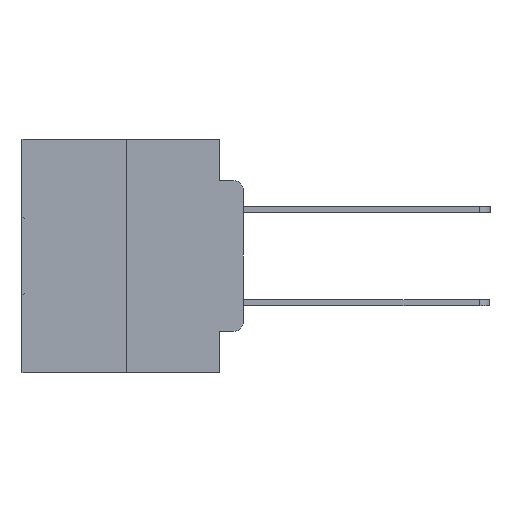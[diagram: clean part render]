
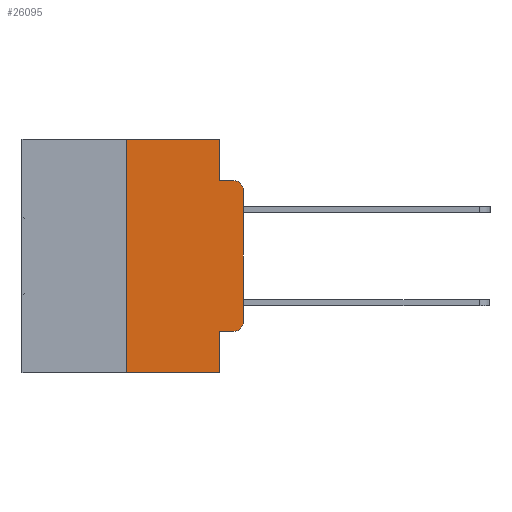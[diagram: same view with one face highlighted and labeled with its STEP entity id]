
A CAD part, left-side view. The second image highlights one B-rep face of the part: STEP entity #26095.
In plain terms, the highlighted planar face has unit normal (-1, 0, 0).
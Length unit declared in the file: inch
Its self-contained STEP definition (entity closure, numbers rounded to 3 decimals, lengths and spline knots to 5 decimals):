
#663 = LINE ( 'NONE', #30555, #26407 ) ;
#740 = ORIENTED_EDGE ( 'NONE', *, *, #30490, .F. ) ;
#1417 = CIRCLE ( 'NONE', #31994, 0.02 ) ;
#1953 = VERTEX_POINT ( 'NONE', #15396 ) ;
#2614 = VERTEX_POINT ( 'NONE', #27927 ) ;
#2710 = ORIENTED_EDGE ( 'NONE', *, *, #6122, .F. ) ;
#2886 = LINE ( 'NONE', #31540, #15412 ) ;
#2908 = VECTOR ( 'NONE', #31604, 39.37008 ) ;
#2981 = VECTOR ( 'NONE', #24101, 39.37008 ) ;
#4121 = EDGE_CURVE ( 'NONE', #15564, #19017, #8856, .T. ) ;
#4308 = DIRECTION ( 'NONE',  ( 1., 0., 0. ) ) ;
#4544 = EDGE_LOOP ( 'NONE', ( #15962, #8123, #16779, #740, #14441, #2710, #28045, #17174, #17570, #15645 ) ) ;
#4629 = LINE ( 'NONE', #19878, #29623 ) ;
#4911 = DIRECTION ( 'NONE',  ( 0., 0., -1. ) ) ;
#5365 = CARTESIAN_POINT ( 'NONE',  ( 0., 0., -0.1085 ) ) ;
#5631 = CARTESIAN_POINT ( 'NONE',  ( 0., 0.25, -0.5 ) ) ;
#6089 = LINE ( 'NONE', #9813, #25972 ) ;
#6122 = EDGE_CURVE ( 'NONE', #10830, #1953, #2886, .T. ) ;
#8123 = ORIENTED_EDGE ( 'NONE', *, *, #11843, .T. ) ;
#8293 = EDGE_CURVE ( 'NONE', #2614, #22981, #23102, .T. ) ;
#8492 = EDGE_CURVE ( 'NONE', #23985, #13070, #17676, .T. ) ;
#8856 = LINE ( 'NONE', #21541, #2981 ) ;
#9065 = CARTESIAN_POINT ( 'NONE',  ( 0., 0.051, 0. ) ) ;
#9229 = CARTESIAN_POINT ( 'NONE',  ( 0., 0.473, 0. ) ) ;
#9553 = DIRECTION ( 'NONE',  ( -1., 0., 0. ) ) ;
#9813 = CARTESIAN_POINT ( 'NONE',  ( 0., 0.473, 0. ) ) ;
#9939 = CARTESIAN_POINT ( 'NONE',  ( 0., 0.02, -0.1085 ) ) ;
#10414 = CIRCLE ( 'NONE', #11865, 0.02 ) ;
#10830 = VERTEX_POINT ( 'NONE', #5631 ) ;
#11491 = EDGE_CURVE ( 'NONE', #10830, #30007, #663, .T. ) ;
#11657 = CARTESIAN_POINT ( 'NONE',  ( 0., 0.051, 0. ) ) ;
#11843 = EDGE_CURVE ( 'NONE', #22981, #19017, #10414, .T. ) ;
#11865 = AXIS2_PLACEMENT_3D ( 'NONE', #9939, #27367, #12462 ) ;
#12462 = DIRECTION ( 'NONE',  ( 0., 0., -1. ) ) ;
#12673 = CARTESIAN_POINT ( 'NONE',  ( 0., 0.051, -0.0885 ) ) ;
#13070 = VERTEX_POINT ( 'NONE', #19602 ) ;
#14263 = PLANE ( 'NONE',  #26954 ) ;
#14441 = ORIENTED_EDGE ( 'NONE', *, *, #20208, .F. ) ;
#14484 = DIRECTION ( 'NONE',  ( 0., 0., 1. ) ) ;
#15396 = CARTESIAN_POINT ( 'NONE',  ( 0., 0.25, 0. ) ) ;
#15412 = VECTOR ( 'NONE', #14484, 39.37008 ) ;
#15564 = VERTEX_POINT ( 'NONE', #12673 ) ;
#15636 = CARTESIAN_POINT ( 'NONE',  ( 0., 0., 0. ) ) ;
#15645 = ORIENTED_EDGE ( 'NONE', *, *, #26149, .T. ) ;
#15962 = ORIENTED_EDGE ( 'NONE', *, *, #8293, .T. ) ;
#16294 = FACE_OUTER_BOUND ( 'NONE', #4544, .T. ) ;
#16779 = ORIENTED_EDGE ( 'NONE', *, *, #4121, .F. ) ;
#17174 = ORIENTED_EDGE ( 'NONE', *, *, #28191, .F. ) ;
#17350 = DIRECTION ( 'NONE',  ( 0., -1., 0. ) ) ;
#17570 = ORIENTED_EDGE ( 'NONE', *, *, #8492, .T. ) ;
#17676 = LINE ( 'NONE', #31849, #30147 ) ;
#18141 = DIRECTION ( 'NONE',  ( 0., -1., 0. ) ) ;
#19017 = VERTEX_POINT ( 'NONE', #29378 ) ;
#19602 = CARTESIAN_POINT ( 'NONE',  ( 0., 0.02, -0.4115 ) ) ;
#19734 = CARTESIAN_POINT ( 'NONE',  ( 0., 0.051, -0.4115 ) ) ;
#19878 = CARTESIAN_POINT ( 'NONE',  ( 0., 0.051, 0. ) ) ;
#20013 = VERTEX_POINT ( 'NONE', #9065 ) ;
#20208 = EDGE_CURVE ( 'NONE', #1953, #20013, #6089, .T. ) ;
#21541 = CARTESIAN_POINT ( 'NONE',  ( 0., 0.051, -0.0885 ) ) ;
#21757 = DIRECTION ( 'NONE',  ( 0., 0., -1. ) ) ;
#22804 = LINE ( 'NONE', #11657, #2908 ) ;
#22981 = VERTEX_POINT ( 'NONE', #5365 ) ;
#23095 = DIRECTION ( 'NONE',  ( 0., 0., 1. ) ) ;
#23102 = LINE ( 'NONE', #15636, #23892 ) ;
#23892 = VECTOR ( 'NONE', #23095, 39.37008 ) ;
#23985 = VERTEX_POINT ( 'NONE', #19734 ) ;
#24101 = DIRECTION ( 'NONE',  ( 0., -1., 0. ) ) ;
#24454 = CARTESIAN_POINT ( 'NONE',  ( 0., 0.02, -0.3915 ) ) ;
#25972 = VECTOR ( 'NONE', #17350, 39.37008 ) ;
#26095 = ADVANCED_FACE ( 'NONE', ( #16294 ), #14263, .F. ) ;
#26149 = EDGE_CURVE ( 'NONE', #13070, #2614, #1417, .T. ) ;
#26407 = VECTOR ( 'NONE', #18141, 39.37008 ) ;
#26816 = DIRECTION ( 'NONE',  ( 0., -1., 0. ) ) ;
#26954 = AXIS2_PLACEMENT_3D ( 'NONE', #9229, #4308, #21757 ) ;
#26979 = DIRECTION ( 'NONE',  ( 0., 0., -1. ) ) ;
#27367 = DIRECTION ( 'NONE',  ( -1., 0., 0. ) ) ;
#27927 = CARTESIAN_POINT ( 'NONE',  ( 0., 0., -0.3915 ) ) ;
#28045 = ORIENTED_EDGE ( 'NONE', *, *, #11491, .T. ) ;
#28191 = EDGE_CURVE ( 'NONE', #23985, #30007, #4629, .T. ) ;
#29378 = CARTESIAN_POINT ( 'NONE',  ( 0., 0.02, -0.0885 ) ) ;
#29623 = VECTOR ( 'NONE', #4911, 39.37008 ) ;
#29795 = CARTESIAN_POINT ( 'NONE',  ( 0., 0.051, -0.5 ) ) ;
#30007 = VERTEX_POINT ( 'NONE', #29795 ) ;
#30147 = VECTOR ( 'NONE', #26816, 39.37008 ) ;
#30490 = EDGE_CURVE ( 'NONE', #20013, #15564, #22804, .T. ) ;
#30555 = CARTESIAN_POINT ( 'NONE',  ( 0., 0.473, -0.5 ) ) ;
#31540 = CARTESIAN_POINT ( 'NONE',  ( 0., 0.25, 0. ) ) ;
#31604 = DIRECTION ( 'NONE',  ( 0., 0., -1. ) ) ;
#31849 = CARTESIAN_POINT ( 'NONE',  ( 0., 0.051, -0.4115 ) ) ;
#31994 = AXIS2_PLACEMENT_3D ( 'NONE', #24454, #9553, #26979 ) ;
